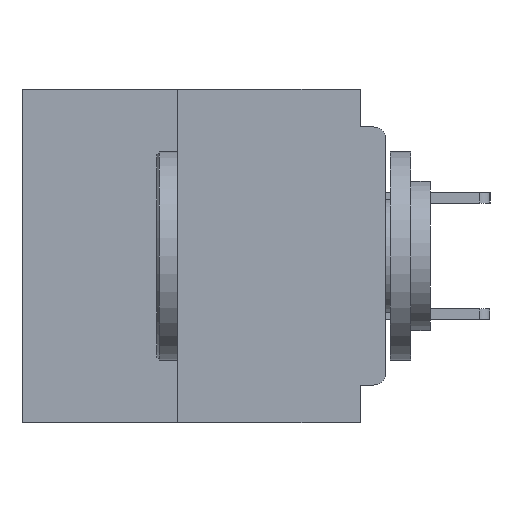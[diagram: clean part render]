
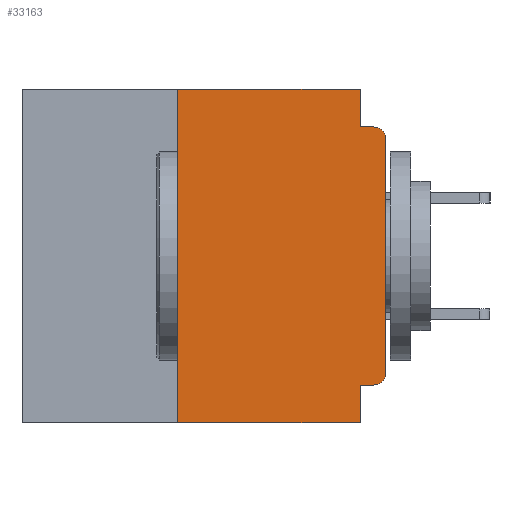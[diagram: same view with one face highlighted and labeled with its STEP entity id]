
A CAD part, left-side view. The second image highlights one B-rep face of the part: STEP entity #33163.
In plain terms, the highlighted planar face has unit normal (-1, 0, 0).
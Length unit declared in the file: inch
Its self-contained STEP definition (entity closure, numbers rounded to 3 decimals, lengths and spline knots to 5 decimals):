
#231 = DIRECTION ( 'NONE',  ( -1., 0., 0. ) ) ;
#1806 = AXIS2_PLACEMENT_3D ( 'NONE', #49808, #20861, #54649 ) ;
#2564 = EDGE_CURVE ( 'NONE', #27295, #18937, #60813, .T. ) ;
#2660 = EDGE_CURVE ( 'NONE', #17119, #18720, #54821, .T. ) ;
#2961 = ORIENTED_EDGE ( 'NONE', *, *, #26310, .F. ) ;
#3087 = CARTESIAN_POINT ( 'NONE',  ( 0., 0., -0.34 ) ) ;
#3755 = ORIENTED_EDGE ( 'NONE', *, *, #60436, .F. ) ;
#4846 = VECTOR ( 'NONE', #12925, 39.37008 ) ;
#5151 = CIRCLE ( 'NONE', #47232, 0.015 ) ;
#5825 = EDGE_LOOP ( 'NONE', ( #9730, #27219, #47503, #2961, #43769, #14626, #41502, #3755, #24419, #52717 ) ) ;
#9730 = ORIENTED_EDGE ( 'NONE', *, *, #2660, .T. ) ;
#9797 = CARTESIAN_POINT ( 'NONE',  ( 0., 0., -0.355 ) ) ;
#11003 = VECTOR ( 'NONE', #21547, 39.37008 ) ;
#11183 = VECTOR ( 'NONE', #27878, 39.37008 ) ;
#11552 = VECTOR ( 'NONE', #13680, 39.37008 ) ;
#11697 = VECTOR ( 'NONE', #37223, 39.37008 ) ;
#11911 = VERTEX_POINT ( 'NONE', #25478 ) ;
#12925 = DIRECTION ( 'NONE',  ( 0., 0., 1. ) ) ;
#12998 = CARTESIAN_POINT ( 'NONE',  ( 0., 0., 0. ) ) ;
#13680 = DIRECTION ( 'NONE',  ( 0., 0., -1. ) ) ;
#14626 = ORIENTED_EDGE ( 'NONE', *, *, #19243, .F. ) ;
#15881 = CARTESIAN_POINT ( 'NONE',  ( 0., 0.031, -0.4 ) ) ;
#15944 = DIRECTION ( 'NONE',  ( 0., -1., 0. ) ) ;
#16233 = EDGE_CURVE ( 'NONE', #18720, #28947, #56288, .T. ) ;
#16290 = CARTESIAN_POINT ( 'NONE',  ( 0., 0.437, 0. ) ) ;
#16643 = CARTESIAN_POINT ( 'NONE',  ( 0., 0.437, -0.4 ) ) ;
#17119 = VERTEX_POINT ( 'NONE', #3087 ) ;
#18720 = VERTEX_POINT ( 'NONE', #46756 ) ;
#18937 = VERTEX_POINT ( 'NONE', #48010 ) ;
#19243 = EDGE_CURVE ( 'NONE', #52774, #27295, #36741, .T. ) ;
#20417 = VECTOR ( 'NONE', #24509, 39.37008 ) ;
#20861 = DIRECTION ( 'NONE',  ( -1., 0., 0. ) ) ;
#21333 = CARTESIAN_POINT ( 'NONE',  ( 0., 0.25, -0.4 ) ) ;
#21468 = EDGE_CURVE ( 'NONE', #52774, #44911, #36841, .T. ) ;
#21547 = DIRECTION ( 'NONE',  ( 0., -1., 0. ) ) ;
#24124 = VERTEX_POINT ( 'NONE', #45492 ) ;
#24419 = ORIENTED_EDGE ( 'NONE', *, *, #47550, .F. ) ;
#24509 = DIRECTION ( 'NONE',  ( 0., 1., 0. ) ) ;
#25478 = CARTESIAN_POINT ( 'NONE',  ( 0., 0.031, -0.045 ) ) ;
#26310 = EDGE_CURVE ( 'NONE', #18937, #11911, #50232, .T. ) ;
#27206 = LINE ( 'NONE', #61576, #11183 ) ;
#27219 = ORIENTED_EDGE ( 'NONE', *, *, #16233, .T. ) ;
#27295 = VERTEX_POINT ( 'NONE', #39768 ) ;
#27878 = DIRECTION ( 'NONE',  ( 0., -1., 0. ) ) ;
#28947 = VERTEX_POINT ( 'NONE', #52673 ) ;
#29341 = CARTESIAN_POINT ( 'NONE',  ( 0., 0.015, -0.34 ) ) ;
#33163 = ADVANCED_FACE ( 'NONE', ( #33351 ), #62411, .F. ) ;
#33314 = LINE ( 'NONE', #9797, #20417 ) ;
#33351 = FACE_OUTER_BOUND ( 'NONE', #5825, .T. ) ;
#33603 = DIRECTION ( 'NONE',  ( 0., 0., -1. ) ) ;
#34203 = DIRECTION ( 'NONE',  ( 0., 0., -1. ) ) ;
#35225 = VECTOR ( 'NONE', #15944, 39.37008 ) ;
#36259 = CARTESIAN_POINT ( 'NONE',  ( 0., 0.015, -0.355 ) ) ;
#36298 = CARTESIAN_POINT ( 'NONE',  ( 0., 0.25, -0.4 ) ) ;
#36741 = LINE ( 'NONE', #21333, #49957 ) ;
#36841 = LINE ( 'NONE', #16643, #11003 ) ;
#37223 = DIRECTION ( 'NONE',  ( 0., 0., -1. ) ) ;
#39561 = AXIS2_PLACEMENT_3D ( 'NONE', #57588, #43087, #33603 ) ;
#39768 = CARTESIAN_POINT ( 'NONE',  ( 0., 0.25, 0. ) ) ;
#40786 = DIRECTION ( 'NONE',  ( 0., 0., 1. ) ) ;
#41502 = ORIENTED_EDGE ( 'NONE', *, *, #21468, .T. ) ;
#43087 = DIRECTION ( 'NONE',  ( 1., 0., 0. ) ) ;
#43769 = ORIENTED_EDGE ( 'NONE', *, *, #2564, .F. ) ;
#44911 = VERTEX_POINT ( 'NONE', #15881 ) ;
#45492 = CARTESIAN_POINT ( 'NONE',  ( 0., 0.031, -0.355 ) ) ;
#46756 = CARTESIAN_POINT ( 'NONE',  ( 0., 0., -0.06 ) ) ;
#47232 = AXIS2_PLACEMENT_3D ( 'NONE', #29341, #231, #34203 ) ;
#47503 = ORIENTED_EDGE ( 'NONE', *, *, #54261, .F. ) ;
#47550 = EDGE_CURVE ( 'NONE', #62091, #24124, #33314, .T. ) ;
#47557 = CARTESIAN_POINT ( 'NONE',  ( 0., 0.031, 0. ) ) ;
#48010 = CARTESIAN_POINT ( 'NONE',  ( 0., 0.031, 0. ) ) ;
#49808 = CARTESIAN_POINT ( 'NONE',  ( 0., 0.015, -0.06 ) ) ;
#49957 = VECTOR ( 'NONE', #40786, 39.37008 ) ;
#50232 = LINE ( 'NONE', #47557, #11552 ) ;
#50373 = LINE ( 'NONE', #61201, #11697 ) ;
#52673 = CARTESIAN_POINT ( 'NONE',  ( 0., 0.015, -0.045 ) ) ;
#52717 = ORIENTED_EDGE ( 'NONE', *, *, #54418, .T. ) ;
#52774 = VERTEX_POINT ( 'NONE', #36298 ) ;
#54261 = EDGE_CURVE ( 'NONE', #11911, #28947, #27206, .T. ) ;
#54418 = EDGE_CURVE ( 'NONE', #62091, #17119, #5151, .T. ) ;
#54649 = DIRECTION ( 'NONE',  ( 0., 0., -1. ) ) ;
#54821 = LINE ( 'NONE', #12998, #4846 ) ;
#56288 = CIRCLE ( 'NONE', #1806, 0.015 ) ;
#57588 = CARTESIAN_POINT ( 'NONE',  ( 0., 0.437, 0. ) ) ;
#60436 = EDGE_CURVE ( 'NONE', #24124, #44911, #50373, .T. ) ;
#60813 = LINE ( 'NONE', #16290, #35225 ) ;
#61201 = CARTESIAN_POINT ( 'NONE',  ( 0., 0.031, -0.4 ) ) ;
#61576 = CARTESIAN_POINT ( 'NONE',  ( 0., 0., -0.045 ) ) ;
#62091 = VERTEX_POINT ( 'NONE', #36259 ) ;
#62411 = PLANE ( 'NONE',  #39561 ) ;
